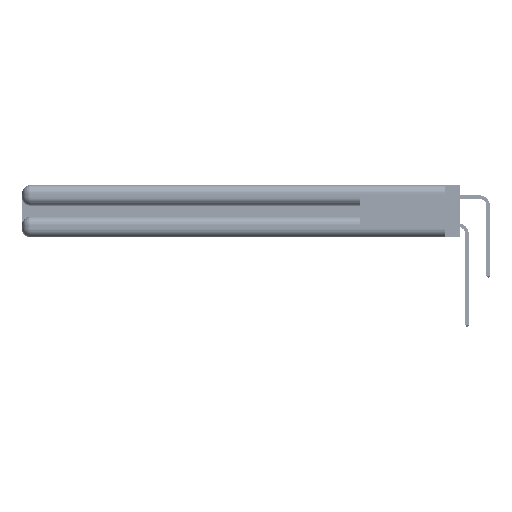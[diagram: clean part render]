
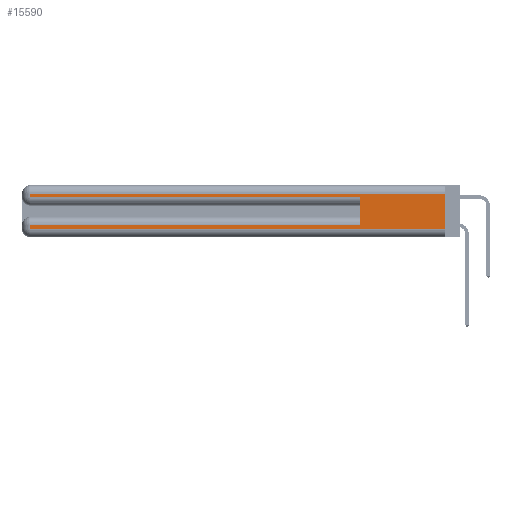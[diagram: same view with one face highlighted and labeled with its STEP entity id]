
A CAD part, left-side view. The second image highlights one B-rep face of the part: STEP entity #15590.
In plain terms, the highlighted planar face has unit normal (-1, 0, 0).
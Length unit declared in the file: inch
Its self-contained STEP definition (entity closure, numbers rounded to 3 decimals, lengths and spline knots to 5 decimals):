
#303 = CARTESIAN_POINT ( 'NONE',  ( 0., 0., 0.31 ) ) ;
#1864 = EDGE_CURVE ( 'NONE', #42718, #30512, #22872, .T. ) ;
#4321 = CARTESIAN_POINT ( 'NONE',  ( 0., 2.94, 0.31 ) ) ;
#6669 = CARTESIAN_POINT ( 'NONE',  ( 0., 2.94, 0.085 ) ) ;
#8376 = ORIENTED_EDGE ( 'NONE', *, *, #22111, .T. ) ;
#13319 = CARTESIAN_POINT ( 'NONE',  ( 0., 0.6, 0.145 ) ) ;
#13425 = VECTOR ( 'NONE', #27750, 39.37008 ) ;
#13926 = EDGE_CURVE ( 'NONE', #21393, #36331, #57862, .T. ) ;
#15590 = ADVANCED_FACE ( 'NONE', ( #20451 ), #28659, .F. ) ;
#16941 = VERTEX_POINT ( 'NONE', #6669 ) ;
#17530 = LINE ( 'NONE', #41436, #57669 ) ;
#18161 = DIRECTION ( 'NONE',  ( 0., 0., 1. ) ) ;
#19142 = VERTEX_POINT ( 'NONE', #50155 ) ;
#20244 = DIRECTION ( 'NONE',  ( 0., 0., -1. ) ) ;
#20451 = FACE_OUTER_BOUND ( 'NONE', #36288, .T. ) ;
#20588 = ORIENTED_EDGE ( 'NONE', *, *, #58285, .T. ) ;
#21393 = VERTEX_POINT ( 'NONE', #42567 ) ;
#22111 = EDGE_CURVE ( 'NONE', #32192, #40744, #34141, .T. ) ;
#22872 = LINE ( 'NONE', #13319, #55083 ) ;
#24605 = LINE ( 'NONE', #303, #51149 ) ;
#24862 = VECTOR ( 'NONE', #25496, 39.37008 ) ;
#25496 = DIRECTION ( 'NONE',  ( 0., 0., -1. ) ) ;
#25701 = CARTESIAN_POINT ( 'NONE',  ( 0., 2.94, 0.285 ) ) ;
#27096 = LINE ( 'NONE', #45784, #13425 ) ;
#27374 = EDGE_CURVE ( 'NONE', #19142, #36331, #54407, .T. ) ;
#27750 = DIRECTION ( 'NONE',  ( 0., 0., -1. ) ) ;
#28659 = PLANE ( 'NONE',  #43847 ) ;
#29058 = EDGE_CURVE ( 'NONE', #16941, #19142, #27096, .T. ) ;
#29256 = DIRECTION ( 'NONE',  ( 0., -1., 0. ) ) ;
#30512 = VERTEX_POINT ( 'NONE', #42982 ) ;
#30642 = DIRECTION ( 'NONE',  ( 0., 0., -1. ) ) ;
#31422 = CARTESIAN_POINT ( 'NONE',  ( 0., 0., 0.37 ) ) ;
#32192 = VERTEX_POINT ( 'NONE', #4321 ) ;
#32377 = EDGE_CURVE ( 'NONE', #40744, #30512, #52689, .T. ) ;
#34141 = LINE ( 'NONE', #43112, #24862 ) ;
#36288 = EDGE_LOOP ( 'NONE', ( #40309, #42055, #8376, #46670, #58079, #20588, #49592, #39743 ) ) ;
#36331 = VERTEX_POINT ( 'NONE', #41082 ) ;
#36820 = DIRECTION ( 'NONE',  ( 0., 1., 0. ) ) ;
#37625 = DIRECTION ( 'NONE',  ( 1., 0., 0. ) ) ;
#39096 = EDGE_CURVE ( 'NONE', #21393, #32192, #24605, .T. ) ;
#39743 = ORIENTED_EDGE ( 'NONE', *, *, #27374, .T. ) ;
#40309 = ORIENTED_EDGE ( 'NONE', *, *, #13926, .F. ) ;
#40744 = VERTEX_POINT ( 'NONE', #25701 ) ;
#41082 = CARTESIAN_POINT ( 'NONE',  ( 0., 0., 0.06 ) ) ;
#41436 = CARTESIAN_POINT ( 'NONE',  ( 0., 0., 0.085 ) ) ;
#42055 = ORIENTED_EDGE ( 'NONE', *, *, #39096, .T. ) ;
#42202 = VECTOR ( 'NONE', #29256, 39.37008 ) ;
#42567 = CARTESIAN_POINT ( 'NONE',  ( 0., 0., 0.31 ) ) ;
#42718 = VERTEX_POINT ( 'NONE', #56137 ) ;
#42846 = CARTESIAN_POINT ( 'NONE',  ( 0., 0., 0.37 ) ) ;
#42982 = CARTESIAN_POINT ( 'NONE',  ( 0., 0.6, 0.285 ) ) ;
#43112 = CARTESIAN_POINT ( 'NONE',  ( 0., 2.94, 0.37 ) ) ;
#43847 = AXIS2_PLACEMENT_3D ( 'NONE', #42846, #37625, #20244 ) ;
#45784 = CARTESIAN_POINT ( 'NONE',  ( 0., 2.94, 0.37 ) ) ;
#46670 = ORIENTED_EDGE ( 'NONE', *, *, #32377, .T. ) ;
#46887 = DIRECTION ( 'NONE',  ( 0., 1., 0. ) ) ;
#47119 = VECTOR ( 'NONE', #30642, 39.37008 ) ;
#49038 = CARTESIAN_POINT ( 'NONE',  ( 0., 0., 0.285 ) ) ;
#49592 = ORIENTED_EDGE ( 'NONE', *, *, #29058, .T. ) ;
#50155 = CARTESIAN_POINT ( 'NONE',  ( 0., 2.94, 0.06 ) ) ;
#51149 = VECTOR ( 'NONE', #46887, 39.37008 ) ;
#51950 = VECTOR ( 'NONE', #56877, 39.37008 ) ;
#52689 = LINE ( 'NONE', #49038, #51950 ) ;
#54407 = LINE ( 'NONE', #56899, #42202 ) ;
#55083 = VECTOR ( 'NONE', #18161, 39.37008 ) ;
#56137 = CARTESIAN_POINT ( 'NONE',  ( 0., 0.6, 0.085 ) ) ;
#56877 = DIRECTION ( 'NONE',  ( 0., -1., 0. ) ) ;
#56899 = CARTESIAN_POINT ( 'NONE',  ( 0., 0., 0.06 ) ) ;
#57669 = VECTOR ( 'NONE', #36820, 39.37008 ) ;
#57862 = LINE ( 'NONE', #31422, #47119 ) ;
#58079 = ORIENTED_EDGE ( 'NONE', *, *, #1864, .F. ) ;
#58285 = EDGE_CURVE ( 'NONE', #42718, #16941, #17530, .T. ) ;
